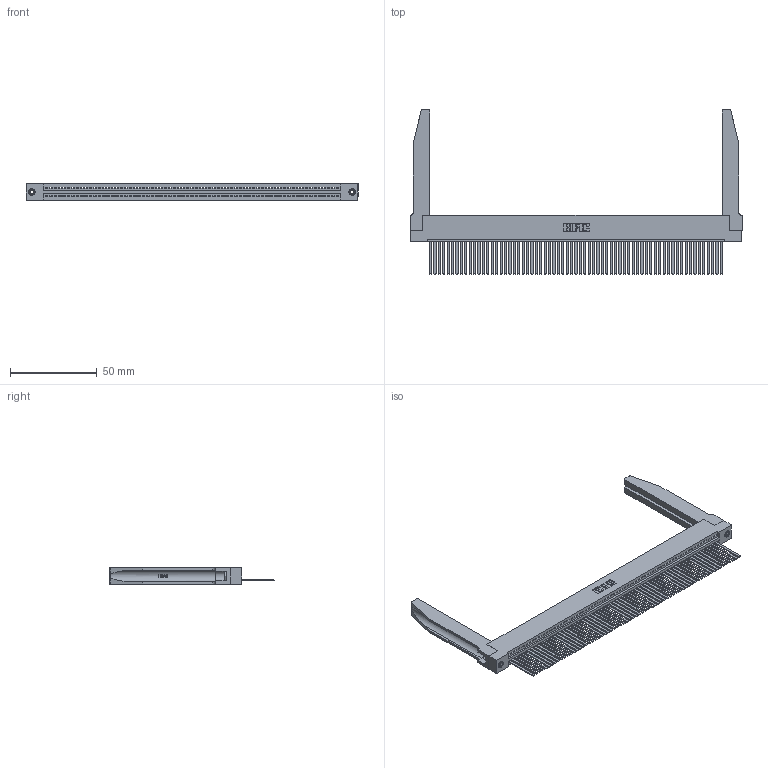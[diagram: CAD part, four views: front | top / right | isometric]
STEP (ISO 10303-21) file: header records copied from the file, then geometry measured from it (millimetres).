
FILE_DESCRIPTION (( 'STEP AP203' ), '1' );
FILE_NAME ('345-067-544-178.STEP', '2019-10-12T03:00:18', ( '' ), ( '' ), 'SwSTEP 2.0', 'SolidWorks 2016', '' );
FILE_SCHEMA (( 'CONFIG_CONTROL_DESIGN' ));
Length unit declared in the file: inch
Products named in the file (5): 345-250-001_345-250-001-102; 345-067-544-178; 345 Part_Flush Mounting Lugs - 0.156 Dia-TH; 345-220-078_345-220-078; 345-292-001_345-293-144
Assembly tree (72 placements, depth 2):
  345-067-544-178
    345 Part_Flush Mounting Lugs - 0.156 Dia-TH
    345-292-001_345-293-144  x67
    345-250-001_345-250-001-102  x2
    345-220-078_345-220-078  x2
Bounding box: 191.41 x 94.92 x 9.4 mm (x, y, z)
Volume: 26932 mm3; surface area: 34978.7 mm2
Topology: 72 solids, 72 shells, 3844 faces, 11535 edges, 7590 vertices
Faces by surface type: plane 2634, cylinder 1158, bspline 36, cone 12, torus 4
Entity records: 51616 total; most frequent: CARTESIAN_POINT 9836, ORIENTED_EDGE 8734, DIRECTION 7559, EDGE_CURVE 4367, VECTOR 3877, LINE 3877, VERTEX_POINT 2904, AXIS2_PLACEMENT_3D 1841
